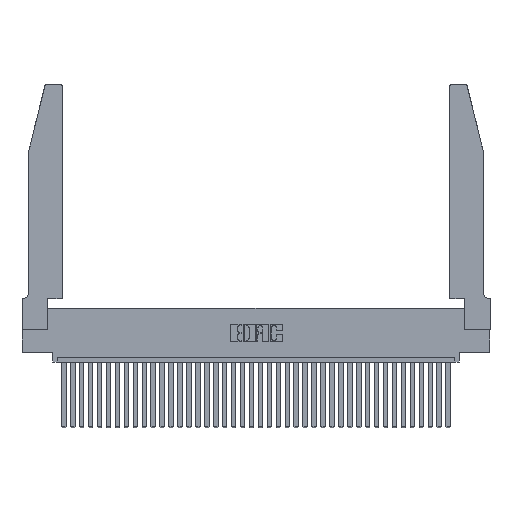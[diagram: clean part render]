
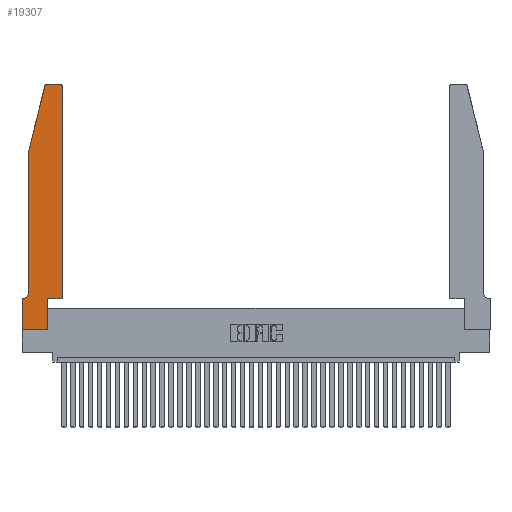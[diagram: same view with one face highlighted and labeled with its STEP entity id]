
A CAD part, top view. The second image highlights one B-rep face of the part: STEP entity #19307.
In plain terms, the highlighted planar face has unit normal (0, 0, 1).
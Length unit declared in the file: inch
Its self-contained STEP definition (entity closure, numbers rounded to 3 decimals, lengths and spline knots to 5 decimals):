
#404 = AXIS2_PLACEMENT_3D ( 'NONE', #35661, #1321, #3686 ) ;
#1159 = CARTESIAN_POINT ( 'NONE',  ( 0.0755, 2., 0.37 ) ) ;
#1321 = DIRECTION ( 'NONE',  ( 0., 0., -1. ) ) ;
#1639 = DIRECTION ( 'NONE',  ( 1., 0., 0. ) ) ;
#2325 = CIRCLE ( 'NONE', #404, 0.07 ) ;
#2482 = ORIENTED_EDGE ( 'NONE', *, *, #12494, .T. ) ;
#3326 = CARTESIAN_POINT ( 'NONE',  ( 0.4505, 0.35, 0.37 ) ) ;
#3374 = DIRECTION ( 'NONE',  ( 1., 0., 0. ) ) ;
#3686 = DIRECTION ( 'NONE',  ( -1., 0., 0. ) ) ;
#3867 = CARTESIAN_POINT ( 'NONE',  ( 0.0755, 2., 0.37 ) ) ;
#3886 = VECTOR ( 'NONE', #21879, 39.37008 ) ;
#5479 = LINE ( 'NONE', #6564, #19570 ) ;
#6058 = AXIS2_PLACEMENT_3D ( 'NONE', #21584, #27562, #1639 ) ;
#6144 = CARTESIAN_POINT ( 'NONE',  ( 0.0755, 2., 0.37 ) ) ;
#6564 = CARTESIAN_POINT ( 'NONE',  ( 0., 0., 0.37 ) ) ;
#6681 = EDGE_CURVE ( 'NONE', #18843, #32423, #13878, .T. ) ;
#6683 = PLANE ( 'NONE',  #19407 ) ;
#6723 = CIRCLE ( 'NONE', #6058, 0.03 ) ;
#6915 = VECTOR ( 'NONE', #26479, 39.37008 ) ;
#7280 = EDGE_CURVE ( 'NONE', #30331, #10717, #16603, .T. ) ;
#7347 = EDGE_CURVE ( 'NONE', #25427, #18843, #23388, .T. ) ;
#7700 = CARTESIAN_POINT ( 'NONE',  ( 0.2865, 0.35, 0.37 ) ) ;
#7788 = VERTEX_POINT ( 'NONE', #3867 ) ;
#8100 = LINE ( 'NONE', #12599, #32169 ) ;
#9496 = ORIENTED_EDGE ( 'NONE', *, *, #15435, .T. ) ;
#9702 = CARTESIAN_POINT ( 'NONE',  ( 0., 0., 0.37 ) ) ;
#9982 = EDGE_CURVE ( 'NONE', #27130, #25427, #5479, .T. ) ;
#10717 = VERTEX_POINT ( 'NONE', #30335 ) ;
#11049 = CARTESIAN_POINT ( 'NONE',  ( 0.0055, 0.35, 0.37 ) ) ;
#11093 = EDGE_CURVE ( 'NONE', #36152, #18035, #6723, .T. ) ;
#11885 = EDGE_LOOP ( 'NONE', ( #16336, #26405, #16417, #2482, #37523, #23202, #9496, #22090, #15123, #17230, #30674, #35367 ) ) ;
#12189 = VECTOR ( 'NONE', #30398, 39.37008 ) ;
#12350 = DIRECTION ( 'NONE',  ( -1., 0., 0. ) ) ;
#12494 = EDGE_CURVE ( 'NONE', #7788, #13901, #20294, .T. ) ;
#12599 = CARTESIAN_POINT ( 'NONE',  ( 0.2605, 2.75, 0.37 ) ) ;
#13080 = LINE ( 'NONE', #23903, #36223 ) ;
#13878 = LINE ( 'NONE', #18568, #15698 ) ;
#13901 = VERTEX_POINT ( 'NONE', #21741 ) ;
#15059 = CARTESIAN_POINT ( 'NONE',  ( 0.284, 2.75, 0.37 ) ) ;
#15075 = CARTESIAN_POINT ( 'NONE',  ( 0.4205, 2.72, 0.37 ) ) ;
#15123 = ORIENTED_EDGE ( 'NONE', *, *, #7347, .T. ) ;
#15435 = EDGE_CURVE ( 'NONE', #30693, #27130, #34313, .T. ) ;
#15698 = VECTOR ( 'NONE', #24532, 39.37008 ) ;
#16336 = ORIENTED_EDGE ( 'NONE', *, *, #29089, .T. ) ;
#16417 = ORIENTED_EDGE ( 'NONE', *, *, #26792, .T. ) ;
#16437 = CARTESIAN_POINT ( 'NONE',  ( 0.4505, 0.35, 0.37 ) ) ;
#16603 = CIRCLE ( 'NONE', #29105, 0.03 ) ;
#17230 = ORIENTED_EDGE ( 'NONE', *, *, #6681, .T. ) ;
#18035 = VERTEX_POINT ( 'NONE', #35491 ) ;
#18568 = CARTESIAN_POINT ( 'NONE',  ( 0.4505, 0.35, 0.37 ) ) ;
#18843 = VERTEX_POINT ( 'NONE', #7700 ) ;
#18917 = VECTOR ( 'NONE', #32884, 39.37008 ) ;
#19031 = CARTESIAN_POINT ( 'NONE',  ( 0.2865, 0.35, 0.37 ) ) ;
#19234 = EDGE_CURVE ( 'NONE', #32423, #30331, #34015, .T. ) ;
#19307 = ADVANCED_FACE ( 'NONE', ( #29023 ), #6683, .T. ) ;
#19407 = AXIS2_PLACEMENT_3D ( 'NONE', #21973, #19667, #21549 ) ;
#19570 = VECTOR ( 'NONE', #3374, 39.37008 ) ;
#19667 = DIRECTION ( 'NONE',  ( 0., 0., 1. ) ) ;
#20294 = LINE ( 'NONE', #1159, #3886 ) ;
#21245 = DIRECTION ( 'NONE',  ( -1., 0., 0. ) ) ;
#21549 = DIRECTION ( 'NONE',  ( 1., 0., 0. ) ) ;
#21584 = CARTESIAN_POINT ( 'NONE',  ( 0.284, 2.72, 0.37 ) ) ;
#21741 = CARTESIAN_POINT ( 'NONE',  ( 0.0755, 0.42, 0.37 ) ) ;
#21879 = DIRECTION ( 'NONE',  ( 0., -1., 0. ) ) ;
#21973 = CARTESIAN_POINT ( 'NONE',  ( 0., 0.35, 0.37 ) ) ;
#22090 = ORIENTED_EDGE ( 'NONE', *, *, #9982, .T. ) ;
#22519 = VECTOR ( 'NONE', #35775, 39.37008 ) ;
#23202 = ORIENTED_EDGE ( 'NONE', *, *, #37490, .T. ) ;
#23388 = LINE ( 'NONE', #19031, #22519 ) ;
#23903 = CARTESIAN_POINT ( 'NONE',  ( 0.0755, 0.35, 0.37 ) ) ;
#24014 = CARTESIAN_POINT ( 'NONE',  ( 0., 0., 0.37 ) ) ;
#24532 = DIRECTION ( 'NONE',  ( 1., 0., 0. ) ) ;
#24834 = CARTESIAN_POINT ( 'NONE',  ( 0.2865, 0., 0.37 ) ) ;
#25427 = VERTEX_POINT ( 'NONE', #24834 ) ;
#26405 = ORIENTED_EDGE ( 'NONE', *, *, #11093, .T. ) ;
#26479 = DIRECTION ( 'NONE',  ( -0.239, -0.971, 0. ) ) ;
#26536 = DIRECTION ( 'NONE',  ( 1., 0., 0. ) ) ;
#26792 = EDGE_CURVE ( 'NONE', #18035, #7788, #32843, .T. ) ;
#26992 = CARTESIAN_POINT ( 'NONE',  ( 0., 0.35, 0.37 ) ) ;
#27130 = VERTEX_POINT ( 'NONE', #9702 ) ;
#27562 = DIRECTION ( 'NONE',  ( 0., 0., 1. ) ) ;
#29023 = FACE_OUTER_BOUND ( 'NONE', #11885, .T. ) ;
#29089 = EDGE_CURVE ( 'NONE', #10717, #36152, #8100, .T. ) ;
#29105 = AXIS2_PLACEMENT_3D ( 'NONE', #15075, #32363, #26536 ) ;
#30331 = VERTEX_POINT ( 'NONE', #33846 ) ;
#30335 = CARTESIAN_POINT ( 'NONE',  ( 0.4205, 2.75, 0.37 ) ) ;
#30398 = DIRECTION ( 'NONE',  ( 0., 1., 0. ) ) ;
#30674 = ORIENTED_EDGE ( 'NONE', *, *, #19234, .T. ) ;
#30693 = VERTEX_POINT ( 'NONE', #26992 ) ;
#32169 = VECTOR ( 'NONE', #12350, 39.37008 ) ;
#32363 = DIRECTION ( 'NONE',  ( 0., 0., 1. ) ) ;
#32423 = VERTEX_POINT ( 'NONE', #3326 ) ;
#32843 = LINE ( 'NONE', #6144, #6915 ) ;
#32884 = DIRECTION ( 'NONE',  ( 0., -1., 0. ) ) ;
#33846 = CARTESIAN_POINT ( 'NONE',  ( 0.4505, 2.72, 0.37 ) ) ;
#34015 = LINE ( 'NONE', #16437, #12189 ) ;
#34313 = LINE ( 'NONE', #24014, #18917 ) ;
#35367 = ORIENTED_EDGE ( 'NONE', *, *, #7280, .T. ) ;
#35491 = CARTESIAN_POINT ( 'NONE',  ( 0.25487, 2.72718, 0.37 ) ) ;
#35551 = EDGE_CURVE ( 'NONE', #13901, #35874, #2325, .T. ) ;
#35661 = CARTESIAN_POINT ( 'NONE',  ( 0.0055, 0.42, 0.37 ) ) ;
#35775 = DIRECTION ( 'NONE',  ( 0., 1., 0. ) ) ;
#35874 = VERTEX_POINT ( 'NONE', #11049 ) ;
#36152 = VERTEX_POINT ( 'NONE', #15059 ) ;
#36223 = VECTOR ( 'NONE', #21245, 39.37008 ) ;
#37490 = EDGE_CURVE ( 'NONE', #35874, #30693, #13080, .T. ) ;
#37523 = ORIENTED_EDGE ( 'NONE', *, *, #35551, .T. ) ;
